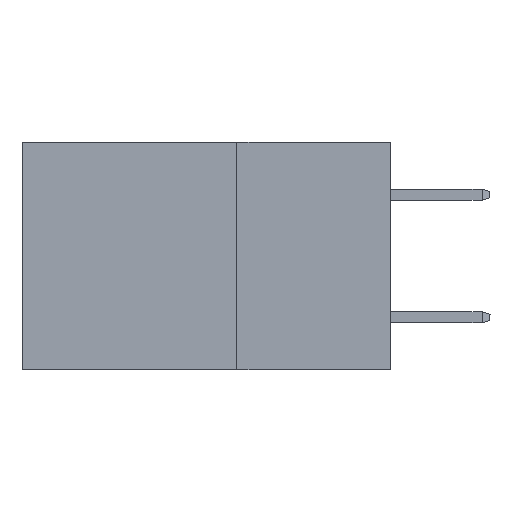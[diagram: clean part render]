
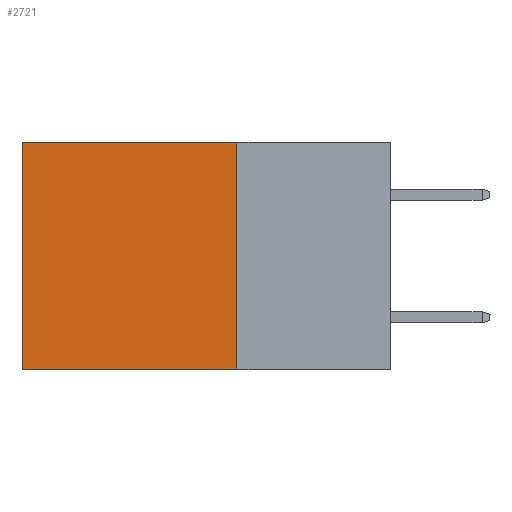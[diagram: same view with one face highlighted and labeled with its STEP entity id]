
A CAD part, left-side view. The second image highlights one B-rep face of the part: STEP entity #2721.
In plain terms, the highlighted planar face has unit normal (-1, 0, 0).
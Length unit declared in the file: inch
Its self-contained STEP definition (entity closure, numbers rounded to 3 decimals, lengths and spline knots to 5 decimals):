
#2721 = ADVANCED_FACE ( 'NONE', ( #39099 ), #23292, .F. ) ;
#2849 = VECTOR ( 'NONE', #18611, 39.37008 ) ;
#3098 = EDGE_CURVE ( 'NONE', #19238, #8816, #16673, .T. ) ;
#4946 = VECTOR ( 'NONE', #8333, 39.37008 ) ;
#5620 = DIRECTION ( 'NONE',  ( 0., 1., 0. ) ) ;
#6013 = LINE ( 'NONE', #7018, #13985 ) ;
#6549 = LINE ( 'NONE', #28709, #4946 ) ;
#6728 = EDGE_CURVE ( 'NONE', #32414, #8816, #6549, .T. ) ;
#7018 = CARTESIAN_POINT ( 'NONE',  ( 0.2875, 0.25, 0. ) ) ;
#8073 = CARTESIAN_POINT ( 'NONE',  ( 0.2875, 0.6, 0. ) ) ;
#8333 = DIRECTION ( 'NONE',  ( 0., 1., 0. ) ) ;
#8816 = VERTEX_POINT ( 'NONE', #33364 ) ;
#9791 = VECTOR ( 'NONE', #5620, 39.37008 ) ;
#12690 = EDGE_CURVE ( 'NONE', #35380, #19238, #21516, .T. ) ;
#13985 = VECTOR ( 'NONE', #24446, 39.37008 ) ;
#14321 = EDGE_CURVE ( 'NONE', #35380, #32414, #6013, .T. ) ;
#16673 = LINE ( 'NONE', #8073, #2849 ) ;
#17712 = CARTESIAN_POINT ( 'NONE',  ( 0.2875, 0.25, 0. ) ) ;
#18611 = DIRECTION ( 'NONE',  ( 0., 0., -1. ) ) ;
#19134 = ORIENTED_EDGE ( 'NONE', *, *, #12690, .T. ) ;
#19192 = CARTESIAN_POINT ( 'NONE',  ( 0.2875, 0.25, 0. ) ) ;
#19238 = VERTEX_POINT ( 'NONE', #22795 ) ;
#21516 = LINE ( 'NONE', #19192, #9791 ) ;
#22795 = CARTESIAN_POINT ( 'NONE',  ( 0.2875, 0.6, 0. ) ) ;
#23292 = PLANE ( 'NONE',  #27546 ) ;
#24446 = DIRECTION ( 'NONE',  ( 0., 0., -1. ) ) ;
#26387 = DIRECTION ( 'NONE',  ( 0., 0., -1. ) ) ;
#27546 = AXIS2_PLACEMENT_3D ( 'NONE', #33654, #37070, #26387 ) ;
#28398 = CARTESIAN_POINT ( 'NONE',  ( 0.2875, 0.25, -0.37 ) ) ;
#28709 = CARTESIAN_POINT ( 'NONE',  ( 0.2875, 0.25, -0.37 ) ) ;
#28803 = EDGE_LOOP ( 'NONE', ( #43206, #36448, #31679, #19134 ) ) ;
#31679 = ORIENTED_EDGE ( 'NONE', *, *, #14321, .F. ) ;
#32414 = VERTEX_POINT ( 'NONE', #28398 ) ;
#33364 = CARTESIAN_POINT ( 'NONE',  ( 0.2875, 0.6, -0.37 ) ) ;
#33654 = CARTESIAN_POINT ( 'NONE',  ( 0.2875, 0.25, 0. ) ) ;
#35380 = VERTEX_POINT ( 'NONE', #17712 ) ;
#36448 = ORIENTED_EDGE ( 'NONE', *, *, #6728, .F. ) ;
#37070 = DIRECTION ( 'NONE',  ( 1., 0., 0. ) ) ;
#39099 = FACE_OUTER_BOUND ( 'NONE', #28803, .T. ) ;
#43206 = ORIENTED_EDGE ( 'NONE', *, *, #3098, .T. ) ;
